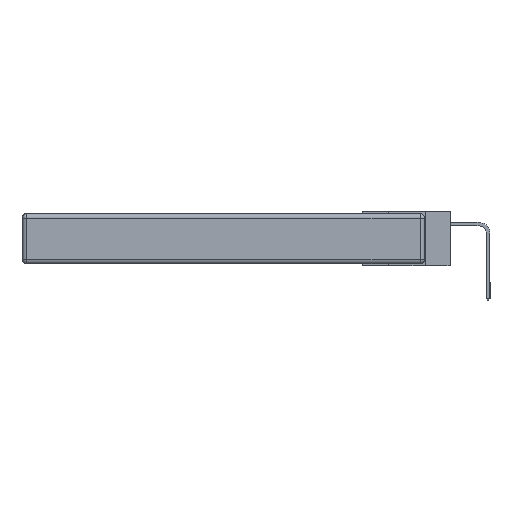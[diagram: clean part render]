
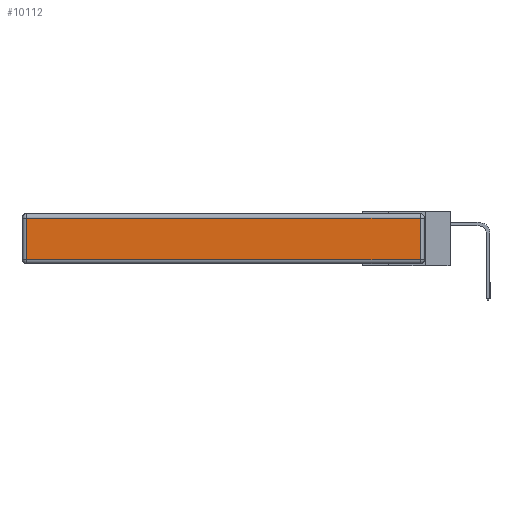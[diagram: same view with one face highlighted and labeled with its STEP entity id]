
A CAD part, left-side view. The second image highlights one B-rep face of the part: STEP entity #10112.
In plain terms, the highlighted planar face has unit normal (-1, 0, 0).
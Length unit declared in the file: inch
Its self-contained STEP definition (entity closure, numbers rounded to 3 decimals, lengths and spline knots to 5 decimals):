
#1288 = CARTESIAN_POINT ( 'NONE',  ( 0., 2.72, -0.343 ) ) ;
#1600 = CARTESIAN_POINT ( 'NONE',  ( 0., 0.03, -0.343 ) ) ;
#3338 = VERTEX_POINT ( 'NONE', #9540 ) ;
#3504 = FACE_OUTER_BOUND ( 'NONE', #16065, .T. ) ;
#3602 = DIRECTION ( 'NONE',  ( 0., 0., 1. ) ) ;
#4473 = VECTOR ( 'NONE', #11220, 39.37008 ) ;
#4647 = DIRECTION ( 'NONE',  ( -1., 0., 0. ) ) ;
#6751 = EDGE_CURVE ( 'NONE', #12034, #9696, #14982, .T. ) ;
#7191 = DIRECTION ( 'NONE',  ( 0., 1., 0. ) ) ;
#7658 = VECTOR ( 'NONE', #21181, 39.37008 ) ;
#8446 = AXIS2_PLACEMENT_3D ( 'NONE', #19313, #4647, #19451 ) ;
#8817 = LINE ( 'NONE', #11363, #4473 ) ;
#9540 = CARTESIAN_POINT ( 'NONE',  ( 0., 2.72, -0.03 ) ) ;
#9696 = VERTEX_POINT ( 'NONE', #15160 ) ;
#10112 = ADVANCED_FACE ( 'NONE', ( #3504 ), #11286, .T. ) ;
#10317 = LINE ( 'NONE', #14013, #16999 ) ;
#10987 = CARTESIAN_POINT ( 'NONE',  ( 0., 2.72, -0.313 ) ) ;
#11220 = DIRECTION ( 'NONE',  ( 0., -1., 0. ) ) ;
#11286 = PLANE ( 'NONE',  #8446 ) ;
#11358 = ORIENTED_EDGE ( 'NONE', *, *, #12569, .T. ) ;
#11363 = CARTESIAN_POINT ( 'NONE',  ( 0., 0., -0.313 ) ) ;
#11953 = CARTESIAN_POINT ( 'NONE',  ( 0., 0.03, -0.313 ) ) ;
#12034 = VERTEX_POINT ( 'NONE', #11953 ) ;
#12569 = EDGE_CURVE ( 'NONE', #16547, #12034, #8817, .T. ) ;
#13403 = EDGE_CURVE ( 'NONE', #9696, #3338, #10317, .T. ) ;
#13895 = LINE ( 'NONE', #1288, #7658 ) ;
#14013 = CARTESIAN_POINT ( 'NONE',  ( 0., 2.75, -0.03 ) ) ;
#14982 = LINE ( 'NONE', #1600, #20616 ) ;
#15033 = EDGE_CURVE ( 'NONE', #3338, #16547, #13895, .T. ) ;
#15160 = CARTESIAN_POINT ( 'NONE',  ( 0., 0.03, -0.03 ) ) ;
#15174 = ORIENTED_EDGE ( 'NONE', *, *, #15033, .T. ) ;
#16065 = EDGE_LOOP ( 'NONE', ( #11358, #18191, #18408, #15174 ) ) ;
#16547 = VERTEX_POINT ( 'NONE', #10987 ) ;
#16999 = VECTOR ( 'NONE', #7191, 39.37008 ) ;
#18191 = ORIENTED_EDGE ( 'NONE', *, *, #6751, .T. ) ;
#18408 = ORIENTED_EDGE ( 'NONE', *, *, #13403, .T. ) ;
#19313 = CARTESIAN_POINT ( 'NONE',  ( 0., 0., -0.343 ) ) ;
#19451 = DIRECTION ( 'NONE',  ( 0., 0., 1. ) ) ;
#20616 = VECTOR ( 'NONE', #3602, 39.37008 ) ;
#21181 = DIRECTION ( 'NONE',  ( 0., 0., -1. ) ) ;
